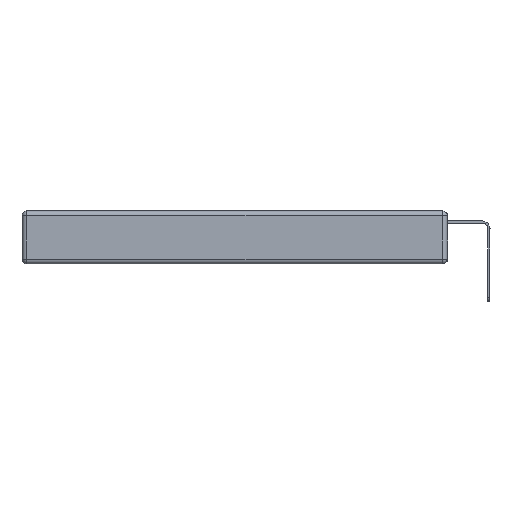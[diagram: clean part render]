
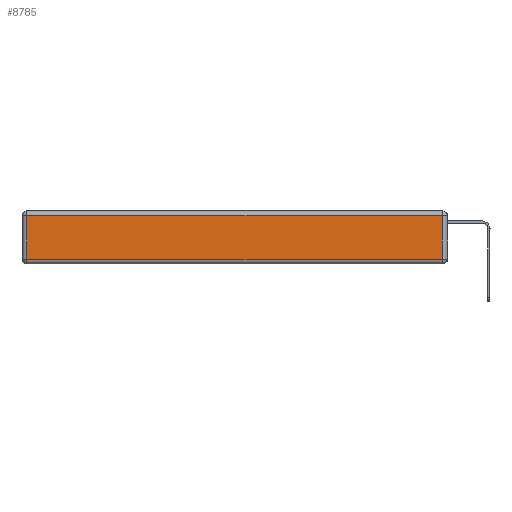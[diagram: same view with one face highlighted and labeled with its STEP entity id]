
A CAD part, left-side view. The second image highlights one B-rep face of the part: STEP entity #8785.
In plain terms, the highlighted planar face has unit normal (-1, 0, 0).
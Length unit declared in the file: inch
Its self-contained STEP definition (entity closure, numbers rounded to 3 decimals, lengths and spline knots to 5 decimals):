
#102 = CARTESIAN_POINT ( 'NONE',  ( 0., 0.03, -0.313 ) ) ;
#520 = CARTESIAN_POINT ( 'NONE',  ( 0., 2.75, -0.03 ) ) ;
#546 = VERTEX_POINT ( 'NONE', #14021 ) ;
#730 = CARTESIAN_POINT ( 'NONE',  ( 0., 2.72, -0.343 ) ) ;
#942 = ORIENTED_EDGE ( 'NONE', *, *, #7182, .T. ) ;
#1257 = CARTESIAN_POINT ( 'NONE',  ( 0., 2.72, -0.313 ) ) ;
#1351 = VERTEX_POINT ( 'NONE', #1257 ) ;
#1417 = CARTESIAN_POINT ( 'NONE',  ( 0., 0., -0.343 ) ) ;
#1455 = DIRECTION ( 'NONE',  ( 0., 0., 1. ) ) ;
#1573 = CARTESIAN_POINT ( 'NONE',  ( 0., 0., -0.313 ) ) ;
#1619 = VECTOR ( 'NONE', #7961, 39.37008 ) ;
#2281 = EDGE_CURVE ( 'NONE', #1351, #4993, #9410, .T. ) ;
#2285 = VECTOR ( 'NONE', #6320, 39.37008 ) ;
#2632 = EDGE_CURVE ( 'NONE', #4993, #12830, #10469, .T. ) ;
#2811 = LINE ( 'NONE', #730, #2285 ) ;
#3250 = EDGE_CURVE ( 'NONE', #12830, #546, #7401, .T. ) ;
#4540 = ORIENTED_EDGE ( 'NONE', *, *, #2632, .T. ) ;
#4993 = VERTEX_POINT ( 'NONE', #102 ) ;
#5246 = ORIENTED_EDGE ( 'NONE', *, *, #3250, .T. ) ;
#5259 = FACE_OUTER_BOUND ( 'NONE', #8307, .T. ) ;
#5680 = AXIS2_PLACEMENT_3D ( 'NONE', #1417, #7066, #1455 ) ;
#6320 = DIRECTION ( 'NONE',  ( 0., 0., -1. ) ) ;
#6394 = VECTOR ( 'NONE', #7237, 39.37008 ) ;
#7066 = DIRECTION ( 'NONE',  ( -1., 0., 0. ) ) ;
#7182 = EDGE_CURVE ( 'NONE', #546, #1351, #2811, .T. ) ;
#7237 = DIRECTION ( 'NONE',  ( 0., -1., 0. ) ) ;
#7401 = LINE ( 'NONE', #520, #10928 ) ;
#7961 = DIRECTION ( 'NONE',  ( 0., 0., 1. ) ) ;
#8307 = EDGE_LOOP ( 'NONE', ( #10522, #4540, #5246, #942 ) ) ;
#8785 = ADVANCED_FACE ( 'NONE', ( #5259 ), #10514, .T. ) ;
#9410 = LINE ( 'NONE', #1573, #6394 ) ;
#10469 = LINE ( 'NONE', #13476, #1619 ) ;
#10514 = PLANE ( 'NONE',  #5680 ) ;
#10522 = ORIENTED_EDGE ( 'NONE', *, *, #2281, .T. ) ;
#10928 = VECTOR ( 'NONE', #12229, 39.37008 ) ;
#12229 = DIRECTION ( 'NONE',  ( 0., 1., 0. ) ) ;
#12830 = VERTEX_POINT ( 'NONE', #13018 ) ;
#13018 = CARTESIAN_POINT ( 'NONE',  ( 0., 0.03, -0.03 ) ) ;
#13476 = CARTESIAN_POINT ( 'NONE',  ( 0., 0.03, -0.343 ) ) ;
#14021 = CARTESIAN_POINT ( 'NONE',  ( 0., 2.72, -0.03 ) ) ;
